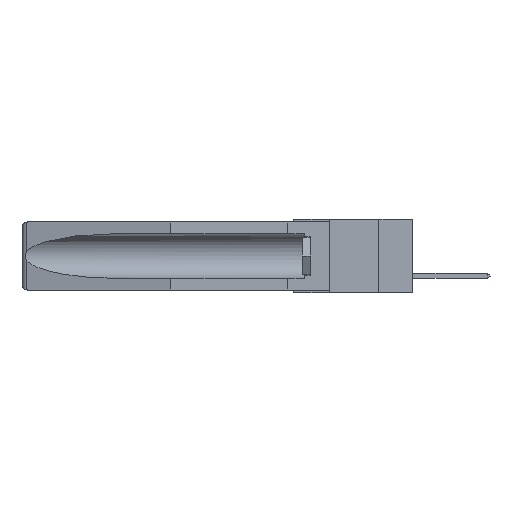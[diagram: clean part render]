
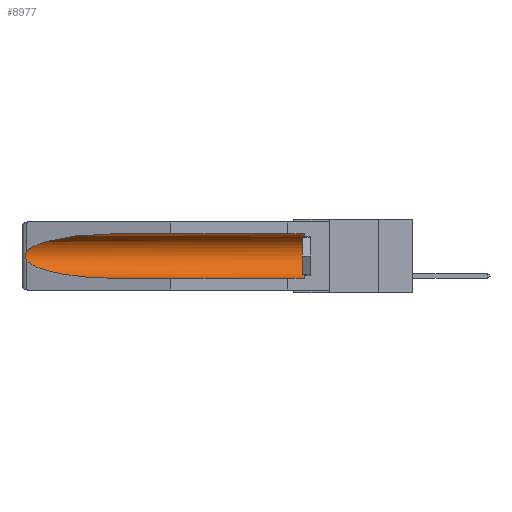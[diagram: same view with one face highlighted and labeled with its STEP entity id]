
A CAD part, left-side view. The second image highlights one B-rep face of the part: STEP entity #8977.
In plain terms, the highlighted cylindrical face has radius 2.857 mm (diameter 5.715 mm), a partial arc.
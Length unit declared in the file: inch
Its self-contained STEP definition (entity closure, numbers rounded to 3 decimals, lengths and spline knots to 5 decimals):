
#73 = CARTESIAN_POINT ( 'NONE',  ( 0.155, 0.126, -0.284 ) ) ;
#488 = CARTESIAN_POINT ( 'NONE',  ( 0.2675, 1.53308, -0.16763 ) ) ;
#583 = DIRECTION ( 'NONE',  ( 0., 0., 1. ) ) ;
#797 = EDGE_CURVE ( 'NONE', #2057, #17381, #9359, .T. ) ;
#2014 = VERTEX_POINT ( 'NONE', #73 ) ;
#2057 = VERTEX_POINT ( 'NONE', #3606 ) ;
#2119 = CARTESIAN_POINT ( 'NONE',  ( 0.26654, 1.53092, -0.15636 ) ) ;
#2259 = EDGE_LOOP ( 'NONE', ( #3810, #15419, #11075, #11447, #14191, #8370 ) ) ;
#2563 = VECTOR ( 'NONE', #4630, 39.37008 ) ;
#3606 = CARTESIAN_POINT ( 'NONE',  ( 0.155, 0.126, -0.059 ) ) ;
#3733 =( BOUNDED_CURVE ( )  B_SPLINE_CURVE ( 3, ( #20632, #10062, #17459, #7055 ),
 .UNSPECIFIED., .F., .F. ) 
 B_SPLINE_CURVE_WITH_KNOTS ( ( 4, 4 ),
 ( 0.1948, 1.5708 ),
 .UNSPECIFIED. ) 
 CURVE ( )  GEOMETRIC_REPRESENTATION_ITEM ( )  RATIONAL_B_SPLINE_CURVE ( ( 1., 0.848, 0.848, 1. ) ) 
 REPRESENTATION_ITEM ( '' )  );
#3773 = CARTESIAN_POINT ( 'NONE',  ( 0.155, -0.30754, -0.1715 ) ) ;
#3810 = ORIENTED_EDGE ( 'NONE', *, *, #13996, .T. ) ;
#4463 = LINE ( 'NONE', #4713, #2563 ) ;
#4630 = DIRECTION ( 'NONE',  ( 0., 1., 0. ) ) ;
#4713 = CARTESIAN_POINT ( 'NONE',  ( 0.155, -0.30754, -0.284 ) ) ;
#4729 =( BOUNDED_CURVE ( )  B_SPLINE_CURVE ( 3, ( #15331, #11765, #17294, #18901 ),
 .UNSPECIFIED., .F., .F. ) 
 B_SPLINE_CURVE_WITH_KNOTS ( ( 4, 4 ),
 ( 4.71239, 6.08839 ),
 .UNSPECIFIED. ) 
 CURVE ( )  GEOMETRIC_REPRESENTATION_ITEM ( )  RATIONAL_B_SPLINE_CURVE ( ( 1., 0.848, 0.848, 1. ) ) 
 REPRESENTATION_ITEM ( '' )  );
#4984 = CYLINDRICAL_SURFACE ( 'NONE', #12115, 0.1125 ) ;
#5559 = CARTESIAN_POINT ( 'NONE',  ( 0.2673, 1.53269, -0.17917 ) ) ;
#7055 = CARTESIAN_POINT ( 'NONE',  ( 0.155, 1.07973, -0.284 ) ) ;
#7168 = FACE_OUTER_BOUND ( 'NONE', #2259, .T. ) ;
#7542 = VERTEX_POINT ( 'NONE', #19323 ) ;
#7554 = AXIS2_PLACEMENT_3D ( 'NONE', #7952, #7805, #583 ) ;
#7805 = DIRECTION ( 'NONE',  ( 0., -1., 0. ) ) ;
#7952 = CARTESIAN_POINT ( 'NONE',  ( 0.155, 0.126, -0.1715 ) ) ;
#8370 = ORIENTED_EDGE ( 'NONE', *, *, #797, .T. ) ;
#8977 = ADVANCED_FACE ( 'NONE', ( #7168 ), #4984, .F. ) ;
#9028 = DIRECTION ( 'NONE',  ( 0., 1., 0. ) ) ;
#9079 = CARTESIAN_POINT ( 'NONE',  ( 0.26597, 1.52961, -0.15275 ) ) ;
#9109 = DIRECTION ( 'NONE',  ( 0., 0., 1. ) ) ;
#9186 = CIRCLE ( 'NONE', #7554, 0.1125 ) ;
#9239 = CARTESIAN_POINT ( 'NONE',  ( 0.26655, 1.53094, -0.18657 ) ) ;
#9359 = LINE ( 'NONE', #15316, #14885 ) ;
#9488 = B_SPLINE_CURVE_WITH_KNOTS ( 'NONE', 3,
 ( #19185, #9079, #2119, #19793, #488, #17876, #5559, #9239, #21496, #14351 ),
 .UNSPECIFIED., .F., .F.,
 ( 4, 2, 2, 2, 4 ),
 ( 0., 0.00029, 0.00058, 0.00087, 0.00117 ),
 .UNSPECIFIED. ) ;
#10062 = CARTESIAN_POINT ( 'NONE',  ( 0.25451, 1.48313, -0.24835 ) ) ;
#11075 = ORIENTED_EDGE ( 'NONE', *, *, #18468, .T. ) ;
#11447 = ORIENTED_EDGE ( 'NONE', *, *, #20180, .F. ) ;
#11765 = CARTESIAN_POINT ( 'NONE',  ( 0.21114, 1.30732, -0.059 ) ) ;
#12115 = AXIS2_PLACEMENT_3D ( 'NONE', #3773, #9028, #9109 ) ;
#12342 = VERTEX_POINT ( 'NONE', #15536 ) ;
#13452 = DIRECTION ( 'NONE',  ( 0., 1., 0. ) ) ;
#13996 = EDGE_CURVE ( 'NONE', #17381, #7542, #4729, .T. ) ;
#14191 = ORIENTED_EDGE ( 'NONE', *, *, #14285, .T. ) ;
#14285 = EDGE_CURVE ( 'NONE', #2014, #2057, #9186, .T. ) ;
#14351 = CARTESIAN_POINT ( 'NONE',  ( 0.26537, 1.52718, -0.19328 ) ) ;
#14885 = VECTOR ( 'NONE', #13452, 39.37008 ) ;
#15044 = VERTEX_POINT ( 'NONE', #20482 ) ;
#15316 = CARTESIAN_POINT ( 'NONE',  ( 0.155, -0.30754, -0.059 ) ) ;
#15331 = CARTESIAN_POINT ( 'NONE',  ( 0.155, 1.07973, -0.059 ) ) ;
#15419 = ORIENTED_EDGE ( 'NONE', *, *, #21023, .T. ) ;
#15536 = CARTESIAN_POINT ( 'NONE',  ( 0.26537, 1.52718, -0.19328 ) ) ;
#16335 = CARTESIAN_POINT ( 'NONE',  ( 0.155, 1.07973, -0.059 ) ) ;
#17294 = CARTESIAN_POINT ( 'NONE',  ( 0.25451, 1.48313, -0.09465 ) ) ;
#17381 = VERTEX_POINT ( 'NONE', #16335 ) ;
#17459 = CARTESIAN_POINT ( 'NONE',  ( 0.21114, 1.30732, -0.284 ) ) ;
#17876 = CARTESIAN_POINT ( 'NONE',  ( 0.2675, 1.53308, -0.17534 ) ) ;
#18468 = EDGE_CURVE ( 'NONE', #12342, #15044, #3733, .T. ) ;
#18901 = CARTESIAN_POINT ( 'NONE',  ( 0.26537, 1.52718, -0.14972 ) ) ;
#19185 = CARTESIAN_POINT ( 'NONE',  ( 0.26537, 1.52718, -0.14972 ) ) ;
#19323 = CARTESIAN_POINT ( 'NONE',  ( 0.26537, 1.52718, -0.14972 ) ) ;
#19793 = CARTESIAN_POINT ( 'NONE',  ( 0.2673, 1.5327, -0.16383 ) ) ;
#20180 = EDGE_CURVE ( 'NONE', #2014, #15044, #4463, .T. ) ;
#20482 = CARTESIAN_POINT ( 'NONE',  ( 0.155, 1.07973, -0.284 ) ) ;
#20632 = CARTESIAN_POINT ( 'NONE',  ( 0.26537, 1.52718, -0.19328 ) ) ;
#21023 = EDGE_CURVE ( 'NONE', #7542, #12342, #9488, .T. ) ;
#21496 = CARTESIAN_POINT ( 'NONE',  ( 0.26597, 1.5296, -0.19026 ) ) ;
